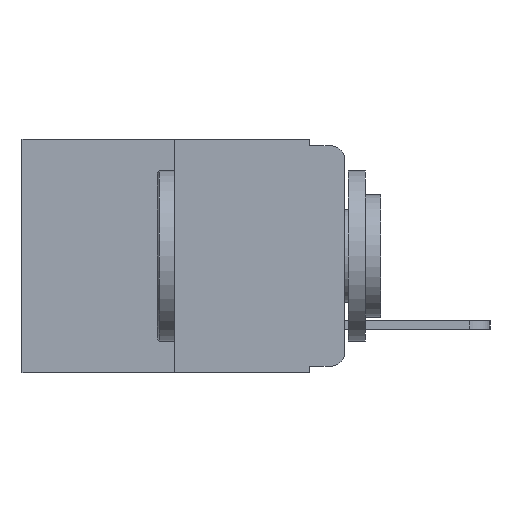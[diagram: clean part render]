
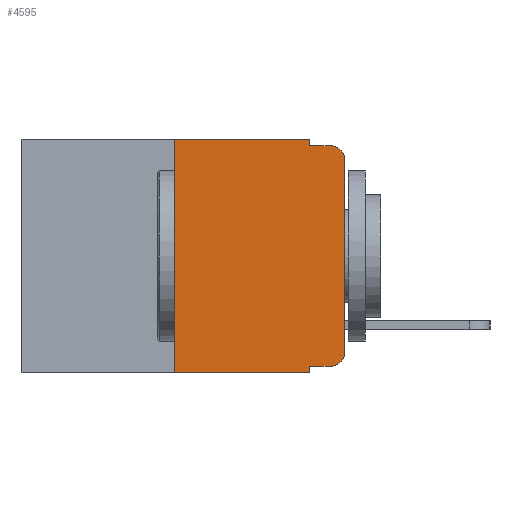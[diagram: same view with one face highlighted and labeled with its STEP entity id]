
A CAD part, left-side view. The second image highlights one B-rep face of the part: STEP entity #4595.
In plain terms, the highlighted planar face has unit normal (-1, 0, 0).
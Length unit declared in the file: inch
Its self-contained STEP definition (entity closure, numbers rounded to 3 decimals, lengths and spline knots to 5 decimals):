
#243 = CARTESIAN_POINT ( 'NONE',  ( 0., 0.051, -0.343 ) ) ;
#1216 = VERTEX_POINT ( 'NONE', #3601 ) ;
#1521 = AXIS2_PLACEMENT_3D ( 'NONE', #6311, #6251, #6240 ) ;
#1531 = AXIS2_PLACEMENT_3D ( 'NONE', #7117, #7104, #7055 ) ;
#1832 = CARTESIAN_POINT ( 'NONE',  ( 0., 0.02, -0.01 ) ) ;
#2378 = ORIENTED_EDGE ( 'NONE', *, *, #12444, .F. ) ;
#2523 = VECTOR ( 'NONE', #6448, 39.37008 ) ;
#3117 = VERTEX_POINT ( 'NONE', #10525 ) ;
#3256 = CARTESIAN_POINT ( 'NONE',  ( 0., 0.051, -0.333 ) ) ;
#3285 = LINE ( 'NONE', #7360, #11475 ) ;
#3601 = CARTESIAN_POINT ( 'NONE',  ( 0., 0., -0.313 ) ) ;
#3895 = ORIENTED_EDGE ( 'NONE', *, *, #12460, .F. ) ;
#3954 = ORIENTED_EDGE ( 'NONE', *, *, #12476, .T. ) ;
#4595 = ADVANCED_FACE ( 'NONE', ( #9412 ), #12733, .F. ) ;
#4952 = VECTOR ( 'NONE', #13045, 39.37008 ) ;
#5235 = CARTESIAN_POINT ( 'NONE',  ( 0., 0.051, -0.01 ) ) ;
#5639 = CIRCLE ( 'NONE', #1521, 0.02 ) ;
#5972 = VECTOR ( 'NONE', #6826, 39.37008 ) ;
#5984 = LINE ( 'NONE', #13646, #4952 ) ;
#6174 = LINE ( 'NONE', #8739, #11318 ) ;
#6240 = DIRECTION ( 'NONE',  ( 0., 0., -1. ) ) ;
#6251 = DIRECTION ( 'NONE',  ( -1., 0., 0. ) ) ;
#6311 = CARTESIAN_POINT ( 'NONE',  ( 0., 0.02, -0.313 ) ) ;
#6344 = VECTOR ( 'NONE', #7582, 39.37008 ) ;
#6408 = DIRECTION ( 'NONE',  ( 0., -1., 0. ) ) ;
#6448 = DIRECTION ( 'NONE',  ( 0., 0., -1. ) ) ;
#6512 = CARTESIAN_POINT ( 'NONE',  ( 0., 0.051, 0. ) ) ;
#6517 = AXIS2_PLACEMENT_3D ( 'NONE', #12098, #12081, #12828 ) ;
#6590 = CARTESIAN_POINT ( 'NONE',  ( 0., 0.25, 0. ) ) ;
#6605 = DIRECTION ( 'NONE',  ( 0., 0., -1. ) ) ;
#6656 = LINE ( 'NONE', #7466, #6344 ) ;
#6774 = CARTESIAN_POINT ( 'NONE',  ( 0., 0.051, -0.333 ) ) ;
#6826 = DIRECTION ( 'NONE',  ( 0., 0., 1. ) ) ;
#6829 = CARTESIAN_POINT ( 'NONE',  ( 0., 0.051, 0. ) ) ;
#6839 = VERTEX_POINT ( 'NONE', #243 ) ;
#7055 = DIRECTION ( 'NONE',  ( 0., 0., -1. ) ) ;
#7104 = DIRECTION ( 'NONE',  ( -1., 0., 0. ) ) ;
#7117 = CARTESIAN_POINT ( 'NONE',  ( 0., 0.02, -0.03 ) ) ;
#7169 = VERTEX_POINT ( 'NONE', #11868 ) ;
#7345 = DIRECTION ( 'NONE',  ( 0., -1., 0. ) ) ;
#7360 = CARTESIAN_POINT ( 'NONE',  ( 0., 0.051, -0.01 ) ) ;
#7466 = CARTESIAN_POINT ( 'NONE',  ( 0., 0., 0. ) ) ;
#7486 = EDGE_LOOP ( 'NONE', ( #8402, #13832, #2378, #3895, #11852, #14363, #8465, #13757, #3954, #8946 ) ) ;
#7582 = DIRECTION ( 'NONE',  ( 0., 0., 1. ) ) ;
#8256 = VERTEX_POINT ( 'NONE', #11370 ) ;
#8346 = DIRECTION ( 'NONE',  ( 0., -1., 0. ) ) ;
#8363 = LINE ( 'NONE', #6512, #2523 ) ;
#8402 = ORIENTED_EDGE ( 'NONE', *, *, #12439, .T. ) ;
#8465 = ORIENTED_EDGE ( 'NONE', *, *, #12245, .T. ) ;
#8675 = LINE ( 'NONE', #6590, #5972 ) ;
#8739 = CARTESIAN_POINT ( 'NONE',  ( 0., 0.473, 0. ) ) ;
#8946 = ORIENTED_EDGE ( 'NONE', *, *, #12480, .T. ) ;
#8982 = VECTOR ( 'NONE', #6605, 39.37008 ) ;
#9412 = FACE_OUTER_BOUND ( 'NONE', #7486, .T. ) ;
#10026 = VERTEX_POINT ( 'NONE', #5235 ) ;
#10406 = VERTEX_POINT ( 'NONE', #1832 ) ;
#10525 = CARTESIAN_POINT ( 'NONE',  ( 0., 0.25, -0.343 ) ) ;
#10742 = VECTOR ( 'NONE', #6408, 39.37008 ) ;
#10784 = VERTEX_POINT ( 'NONE', #11074 ) ;
#11074 = CARTESIAN_POINT ( 'NONE',  ( 0., 0.02, -0.333 ) ) ;
#11122 = LINE ( 'NONE', #6774, #10742 ) ;
#11318 = VECTOR ( 'NONE', #8346, 39.37008 ) ;
#11370 = CARTESIAN_POINT ( 'NONE',  ( 0., 0.25, 0. ) ) ;
#11475 = VECTOR ( 'NONE', #7345, 39.37008 ) ;
#11556 = VERTEX_POINT ( 'NONE', #3256 ) ;
#11787 = CIRCLE ( 'NONE', #1531, 0.02 ) ;
#11852 = ORIENTED_EDGE ( 'NONE', *, *, #12032, .F. ) ;
#11868 = CARTESIAN_POINT ( 'NONE',  ( 0., 0., -0.03 ) ) ;
#12032 = EDGE_CURVE ( 'NONE', #8256, #14069, #6174, .T. ) ;
#12081 = DIRECTION ( 'NONE',  ( 1., 0., 0. ) ) ;
#12098 = CARTESIAN_POINT ( 'NONE',  ( 0., 0.473, 0. ) ) ;
#12245 = EDGE_CURVE ( 'NONE', #3117, #6839, #5984, .T. ) ;
#12439 = EDGE_CURVE ( 'NONE', #1216, #7169, #6656, .T. ) ;
#12440 = EDGE_CURVE ( 'NONE', #7169, #10406, #11787, .T. ) ;
#12444 = EDGE_CURVE ( 'NONE', #10026, #10406, #3285, .T. ) ;
#12460 = EDGE_CURVE ( 'NONE', #14069, #10026, #14089, .T. ) ;
#12463 = EDGE_CURVE ( 'NONE', #3117, #8256, #8675, .T. ) ;
#12464 = EDGE_CURVE ( 'NONE', #11556, #6839, #8363, .T. ) ;
#12476 = EDGE_CURVE ( 'NONE', #11556, #10784, #11122, .T. ) ;
#12480 = EDGE_CURVE ( 'NONE', #10784, #1216, #5639, .T. ) ;
#12733 = PLANE ( 'NONE',  #6517 ) ;
#12828 = DIRECTION ( 'NONE',  ( 0., 0., -1. ) ) ;
#13045 = DIRECTION ( 'NONE',  ( 0., -1., 0. ) ) ;
#13170 = CARTESIAN_POINT ( 'NONE',  ( 0., 0.051, 0. ) ) ;
#13646 = CARTESIAN_POINT ( 'NONE',  ( 0., 0.473, -0.343 ) ) ;
#13757 = ORIENTED_EDGE ( 'NONE', *, *, #12464, .F. ) ;
#13832 = ORIENTED_EDGE ( 'NONE', *, *, #12440, .T. ) ;
#14069 = VERTEX_POINT ( 'NONE', #13170 ) ;
#14089 = LINE ( 'NONE', #6829, #8982 ) ;
#14363 = ORIENTED_EDGE ( 'NONE', *, *, #12463, .F. ) ;
